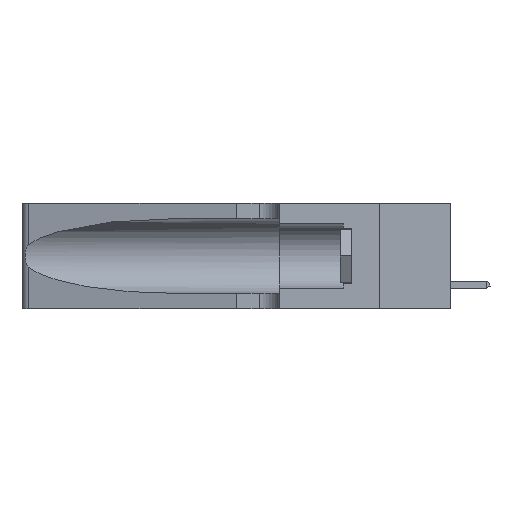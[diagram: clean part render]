
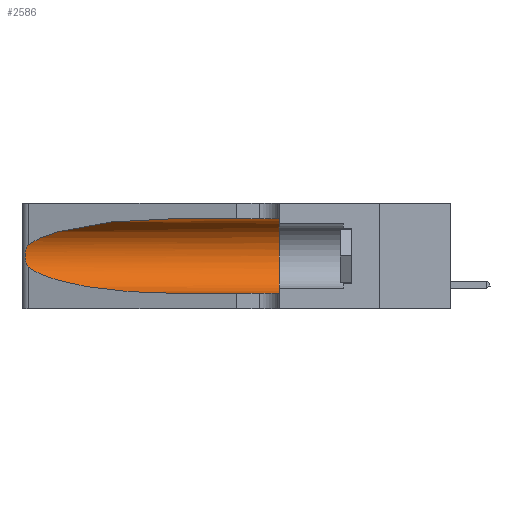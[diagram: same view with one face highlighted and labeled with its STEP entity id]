
A CAD part, left-side view. The second image highlights one B-rep face of the part: STEP entity #2586.
In plain terms, the highlighted cylindrical face has radius 3.308 mm (diameter 6.617 mm), a partial arc.
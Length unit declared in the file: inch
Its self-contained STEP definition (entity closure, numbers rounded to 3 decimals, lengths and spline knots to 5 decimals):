
#443 = DIRECTION ( 'NONE',  ( 0., -1., 0. ) ) ;
#488 = CARTESIAN_POINT ( 'NONE',  ( 0.1305, 1.61858, 0.05475 ) ) ;
#639 = CARTESIAN_POINT ( 'NONE',  ( 0.1305, 0.35, 0.31525 ) ) ;
#2586 = ADVANCED_FACE ( 'NONE', ( #19701 ), #9297, .F. ) ;
#2718 = EDGE_CURVE ( 'NONE', #37705, #10304, #24384, .T. ) ;
#3199 =( BOUNDED_CURVE ( )  B_SPLINE_CURVE ( 3, ( #11771, #4804, #35049, #8008 ),
 .UNSPECIFIED., .F., .F. ) 
 B_SPLINE_CURVE_WITH_KNOTS ( ( 4, 4 ),
 ( 1.5708, 2.84003 ),
 .UNSPECIFIED. ) 
 CURVE ( )  GEOMETRIC_REPRESENTATION_ITEM ( )  RATIONAL_B_SPLINE_CURVE ( ( 1., 0.87, 0.87, 1. ) ) 
 REPRESENTATION_ITEM ( '' )  );
#4804 = CARTESIAN_POINT ( 'NONE',  ( 0.18966, 0.96281, 0.31525 ) ) ;
#5969 = CARTESIAN_POINT ( 'NONE',  ( 0.25487, 1.22718, 0.14631 ) ) ;
#8008 = CARTESIAN_POINT ( 'NONE',  ( 0.25487, 1.22718, 0.22369 ) ) ;
#8492 = ORIENTED_EDGE ( 'NONE', *, *, #31806, .T. ) ;
#9137 = VERTEX_POINT ( 'NONE', #40270 ) ;
#9297 = CYLINDRICAL_SURFACE ( 'NONE', #39667, 0.13025 ) ;
#10022 = ORIENTED_EDGE ( 'NONE', *, *, #21861, .F. ) ;
#10198 = EDGE_CURVE ( 'NONE', #18269, #42011, #10940, .T. ) ;
#10304 = VERTEX_POINT ( 'NONE', #639 ) ;
#10792 = CARTESIAN_POINT ( 'NONE',  ( 0.25487, 1.22718, 0.14631 ) ) ;
#10940 = B_SPLINE_CURVE_WITH_KNOTS ( 'NONE', 3,
 ( #20123, #12978, #33201, #39870, #13270, #36555, #39595, #23050, #36842, #16941, #23332, #23476, #30118, #19692 ),
 .UNSPECIFIED., .F., .F.,
 ( 4, 2, 2, 2, 2, 2, 4 ),
 ( 0., 0.00027, 0.00053, 0.00107, 0.0016, 0.00187, 0.00214 ),
 .UNSPECIFIED. ) ;
#11771 = CARTESIAN_POINT ( 'NONE',  ( 0.1305, 0.72297, 0.31525 ) ) ;
#12801 = CARTESIAN_POINT ( 'NONE',  ( 0.1305, 0.72297, 0.05475 ) ) ;
#12978 = CARTESIAN_POINT ( 'NONE',  ( 0.25555, 1.22994, 0.2215 ) ) ;
#13270 = CARTESIAN_POINT ( 'NONE',  ( 0.25854, 1.2359, 0.20912 ) ) ;
#15555 = CIRCLE ( 'NONE', #32189, 0.13025 ) ;
#16240 = VECTOR ( 'NONE', #23756, 39.37008 ) ;
#16320 = CARTESIAN_POINT ( 'NONE',  ( 0.2373, 1.15595, 0.08982 ) ) ;
#16941 = CARTESIAN_POINT ( 'NONE',  ( 0.25856, 1.23593, 0.16098 ) ) ;
#18269 = VERTEX_POINT ( 'NONE', #29252 ) ;
#19692 = CARTESIAN_POINT ( 'NONE',  ( 0.25487, 1.22718, 0.14631 ) ) ;
#19701 = FACE_OUTER_BOUND ( 'NONE', #27199, .T. ) ;
#19890 = DIRECTION ( 'NONE',  ( 0., 1., 0. ) ) ;
#20006 = DIRECTION ( 'NONE',  ( 0., 0., -1. ) ) ;
#20123 = CARTESIAN_POINT ( 'NONE',  ( 0.25487, 1.22718, 0.22369 ) ) ;
#21831 = VERTEX_POINT ( 'NONE', #32971 ) ;
#21861 = EDGE_CURVE ( 'NONE', #10304, #9137, #15555, .T. ) ;
#22452 = LINE ( 'NONE', #488, #16240 ) ;
#22510 = ORIENTED_EDGE ( 'NONE', *, *, #31210, .T. ) ;
#23050 = CARTESIAN_POINT ( 'NONE',  ( 0.26075, 1.23896, 0.178 ) ) ;
#23332 = CARTESIAN_POINT ( 'NONE',  ( 0.25789, 1.23486, 0.15765 ) ) ;
#23476 = CARTESIAN_POINT ( 'NONE',  ( 0.25639, 1.23186, 0.15144 ) ) ;
#23756 = DIRECTION ( 'NONE',  ( 0., -1., 0. ) ) ;
#24223 = ORIENTED_EDGE ( 'NONE', *, *, #10198, .T. ) ;
#24384 = LINE ( 'NONE', #37231, #31654 ) ;
#26213 = CARTESIAN_POINT ( 'NONE',  ( 0.18966, 0.96281, 0.05475 ) ) ;
#27199 = EDGE_LOOP ( 'NONE', ( #8492, #24223, #32963, #22510, #10022, #30909 ) ) ;
#29252 = CARTESIAN_POINT ( 'NONE',  ( 0.25487, 1.22718, 0.22369 ) ) ;
#29873 = CARTESIAN_POINT ( 'NONE',  ( 0.1305, 1.61858, 0.185 ) ) ;
#30118 = CARTESIAN_POINT ( 'NONE',  ( 0.25555, 1.22993, 0.14849 ) ) ;
#30909 = ORIENTED_EDGE ( 'NONE', *, *, #2718, .F. ) ;
#30930 =( BOUNDED_CURVE ( )  B_SPLINE_CURVE ( 3, ( #5969, #16320, #26213, #12801 ),
 .UNSPECIFIED., .F., .F. ) 
 B_SPLINE_CURVE_WITH_KNOTS ( ( 4, 4 ),
 ( 3.44316, 4.71239 ),
 .UNSPECIFIED. ) 
 CURVE ( )  GEOMETRIC_REPRESENTATION_ITEM ( )  RATIONAL_B_SPLINE_CURVE ( ( 1., 0.87, 0.87, 1. ) ) 
 REPRESENTATION_ITEM ( '' )  );
#31210 = EDGE_CURVE ( 'NONE', #21831, #9137, #22452, .T. ) ;
#31654 = VECTOR ( 'NONE', #443, 39.37008 ) ;
#31806 = EDGE_CURVE ( 'NONE', #37705, #18269, #3199, .T. ) ;
#32189 = AXIS2_PLACEMENT_3D ( 'NONE', #36754, #19890, #42843 ) ;
#32598 = EDGE_CURVE ( 'NONE', #42011, #21831, #30930, .T. ) ;
#32963 = ORIENTED_EDGE ( 'NONE', *, *, #32598, .T. ) ;
#32971 = CARTESIAN_POINT ( 'NONE',  ( 0.1305, 0.72297, 0.05475 ) ) ;
#33201 = CARTESIAN_POINT ( 'NONE',  ( 0.25639, 1.23184, 0.21858 ) ) ;
#35049 = CARTESIAN_POINT ( 'NONE',  ( 0.2373, 1.15595, 0.28018 ) ) ;
#36200 = CARTESIAN_POINT ( 'NONE',  ( 0.1305, 0.72297, 0.31525 ) ) ;
#36555 = CARTESIAN_POINT ( 'NONE',  ( 0.26018, 1.23835, 0.19895 ) ) ;
#36754 = CARTESIAN_POINT ( 'NONE',  ( 0.1305, 0.35, 0.185 ) ) ;
#36842 = CARTESIAN_POINT ( 'NONE',  ( 0.26017, 1.23833, 0.17102 ) ) ;
#37231 = CARTESIAN_POINT ( 'NONE',  ( 0.1305, 1.61858, 0.31525 ) ) ;
#37705 = VERTEX_POINT ( 'NONE', #36200 ) ;
#39595 = CARTESIAN_POINT ( 'NONE',  ( 0.26075, 1.23896, 0.19203 ) ) ;
#39667 = AXIS2_PLACEMENT_3D ( 'NONE', #29873, #39903, #20006 ) ;
#39870 = CARTESIAN_POINT ( 'NONE',  ( 0.25787, 1.23484, 0.2124 ) ) ;
#39903 = DIRECTION ( 'NONE',  ( 0., -1., 0. ) ) ;
#40270 = CARTESIAN_POINT ( 'NONE',  ( 0.1305, 0.35, 0.05475 ) ) ;
#42011 = VERTEX_POINT ( 'NONE', #10792 ) ;
#42843 = DIRECTION ( 'NONE',  ( 0., 0., 1. ) ) ;
